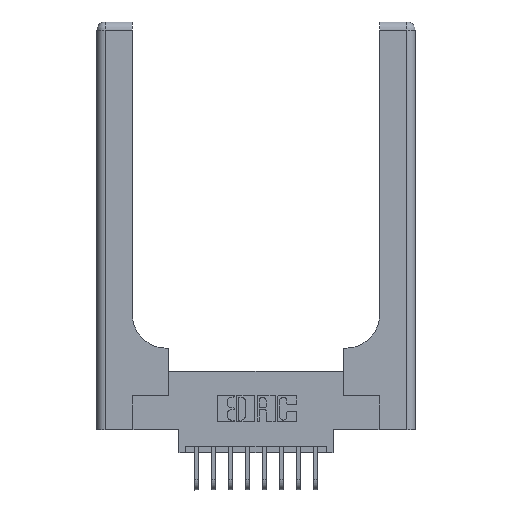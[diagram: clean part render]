
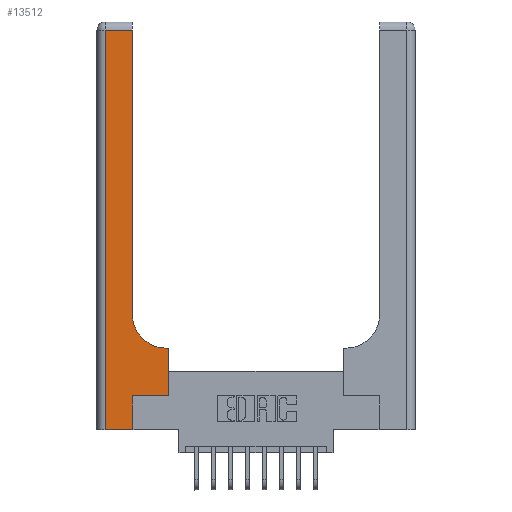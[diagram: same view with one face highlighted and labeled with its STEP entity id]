
A CAD part, top view. The second image highlights one B-rep face of the part: STEP entity #13512.
In plain terms, the highlighted planar face has unit normal (0, 0, 1).
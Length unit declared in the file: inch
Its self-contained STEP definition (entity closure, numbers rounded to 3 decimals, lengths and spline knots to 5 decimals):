
#65 = ORIENTED_EDGE ( 'NONE', *, *, #917, .T. ) ;
#522 = CARTESIAN_POINT ( 'NONE',  ( 0.265, 0., 0.37 ) ) ;
#796 = CIRCLE ( 'NONE', #4579, 0.25 ) ;
#917 = EDGE_CURVE ( 'NONE', #2064, #16770, #10109, .T. ) ;
#1860 = CARTESIAN_POINT ( 'NONE',  ( 0.26, 0.6, 0.37 ) ) ;
#1977 = CARTESIAN_POINT ( 'NONE',  ( 0.26, 2.94, 0.37 ) ) ;
#2064 = VERTEX_POINT ( 'NONE', #3688 ) ;
#2270 = DIRECTION ( 'NONE',  ( 1., 0., 0. ) ) ;
#2379 = EDGE_CURVE ( 'NONE', #6784, #4947, #11821, .T. ) ;
#2435 = DIRECTION ( 'NONE',  ( 0., -1., 0. ) ) ;
#2503 = ORIENTED_EDGE ( 'NONE', *, *, #14546, .T. ) ;
#2571 = CARTESIAN_POINT ( 'NONE',  ( 0.51, 0.85, 0.37 ) ) ;
#2662 = LINE ( 'NONE', #3938, #7397 ) ;
#2764 = CARTESIAN_POINT ( 'NONE',  ( 0., 2.94, 0.37 ) ) ;
#3025 = LINE ( 'NONE', #16448, #16557 ) ;
#3274 = ORIENTED_EDGE ( 'NONE', *, *, #13475, .T. ) ;
#3479 = VECTOR ( 'NONE', #13359, 39.37008 ) ;
#3624 = VERTEX_POINT ( 'NONE', #9985 ) ;
#3656 = ORIENTED_EDGE ( 'NONE', *, *, #9243, .T. ) ;
#3688 = CARTESIAN_POINT ( 'NONE',  ( 0.06, 2.94, 0.37 ) ) ;
#3707 = PLANE ( 'NONE',  #10361 ) ;
#3938 = CARTESIAN_POINT ( 'NONE',  ( 0., 0., 0.37 ) ) ;
#4246 = CARTESIAN_POINT ( 'NONE',  ( 0.26, 0.85, 0.37 ) ) ;
#4528 = EDGE_CURVE ( 'NONE', #3624, #11005, #8573, .T. ) ;
#4579 = AXIS2_PLACEMENT_3D ( 'NONE', #2571, #7801, #2270 ) ;
#4947 = VERTEX_POINT ( 'NONE', #10256 ) ;
#5030 = CARTESIAN_POINT ( 'NONE',  ( 0.06, 0., 0.37 ) ) ;
#5054 = DIRECTION ( 'NONE',  ( 0., 0., -1. ) ) ;
#5061 = VERTEX_POINT ( 'NONE', #11224 ) ;
#5153 = DIRECTION ( 'NONE',  ( -1., 0., 0. ) ) ;
#5230 = VERTEX_POINT ( 'NONE', #1977 ) ;
#6205 = ORIENTED_EDGE ( 'NONE', *, *, #16440, .T. ) ;
#6784 = VERTEX_POINT ( 'NONE', #522 ) ;
#7018 = LINE ( 'NONE', #12046, #3479 ) ;
#7397 = VECTOR ( 'NONE', #10463, 39.37008 ) ;
#7555 = ORIENTED_EDGE ( 'NONE', *, *, #4528, .T. ) ;
#7801 = DIRECTION ( 'NONE',  ( 0., 0., -1. ) ) ;
#7828 = CARTESIAN_POINT ( 'NONE',  ( 0.06, 3., 0.37 ) ) ;
#7965 = VECTOR ( 'NONE', #10475, 39.37008 ) ;
#8277 = EDGE_CURVE ( 'NONE', #5061, #3624, #7018, .T. ) ;
#8435 = CARTESIAN_POINT ( 'NONE',  ( 0.26, 3., 0.37 ) ) ;
#8573 = LINE ( 'NONE', #1860, #15773 ) ;
#9066 = ORIENTED_EDGE ( 'NONE', *, *, #8277, .T. ) ;
#9243 = EDGE_CURVE ( 'NONE', #11005, #11994, #796, .T. ) ;
#9248 = EDGE_LOOP ( 'NONE', ( #2503, #6205, #65, #13082, #15796, #3274, #9066, #7555, #3656 ) ) ;
#9613 = FACE_OUTER_BOUND ( 'NONE', #9248, .T. ) ;
#9985 = CARTESIAN_POINT ( 'NONE',  ( 0.528, 0.6, 0.37 ) ) ;
#10109 = LINE ( 'NONE', #7828, #13998 ) ;
#10256 = CARTESIAN_POINT ( 'NONE',  ( 0.265, 0.25, 0.37 ) ) ;
#10361 = AXIS2_PLACEMENT_3D ( 'NONE', #11624, #5054, #5153 ) ;
#10463 = DIRECTION ( 'NONE',  ( 1., 0., 0. ) ) ;
#10475 = DIRECTION ( 'NONE',  ( 0., 1., 0. ) ) ;
#11005 = VERTEX_POINT ( 'NONE', #15012 ) ;
#11224 = CARTESIAN_POINT ( 'NONE',  ( 0.528, 0.25, 0.37 ) ) ;
#11227 = DIRECTION ( 'NONE',  ( 0., 1., 0. ) ) ;
#11624 = CARTESIAN_POINT ( 'NONE',  ( 0., 3., 0.37 ) ) ;
#11821 = LINE ( 'NONE', #14275, #7965 ) ;
#11921 = VECTOR ( 'NONE', #11227, 39.37008 ) ;
#11994 = VERTEX_POINT ( 'NONE', #4246 ) ;
#12046 = CARTESIAN_POINT ( 'NONE',  ( 0.528, 0.25, 0.37 ) ) ;
#12271 = LINE ( 'NONE', #8435, #11921 ) ;
#12377 = DIRECTION ( 'NONE',  ( -1., 0., 0. ) ) ;
#12461 = LINE ( 'NONE', #2764, #14900 ) ;
#13082 = ORIENTED_EDGE ( 'NONE', *, *, #13214, .T. ) ;
#13190 = DIRECTION ( 'NONE',  ( -1., 0., 0. ) ) ;
#13214 = EDGE_CURVE ( 'NONE', #16770, #6784, #2662, .T. ) ;
#13359 = DIRECTION ( 'NONE',  ( 0., 1., 0. ) ) ;
#13475 = EDGE_CURVE ( 'NONE', #4947, #5061, #3025, .T. ) ;
#13512 = ADVANCED_FACE ( 'NONE', ( #9613 ), #3707, .F. ) ;
#13998 = VECTOR ( 'NONE', #2435, 39.37008 ) ;
#14275 = CARTESIAN_POINT ( 'NONE',  ( 0.265, 0., 0.37 ) ) ;
#14546 = EDGE_CURVE ( 'NONE', #11994, #5230, #12271, .T. ) ;
#14900 = VECTOR ( 'NONE', #13190, 39.37008 ) ;
#15012 = CARTESIAN_POINT ( 'NONE',  ( 0.51, 0.6, 0.37 ) ) ;
#15773 = VECTOR ( 'NONE', #12377, 39.37008 ) ;
#15796 = ORIENTED_EDGE ( 'NONE', *, *, #2379, .T. ) ;
#16440 = EDGE_CURVE ( 'NONE', #5230, #2064, #12461, .T. ) ;
#16448 = CARTESIAN_POINT ( 'NONE',  ( 0.265, 0.25, 0.37 ) ) ;
#16552 = DIRECTION ( 'NONE',  ( 1., 0., 0. ) ) ;
#16557 = VECTOR ( 'NONE', #16552, 39.37008 ) ;
#16770 = VERTEX_POINT ( 'NONE', #5030 ) ;
